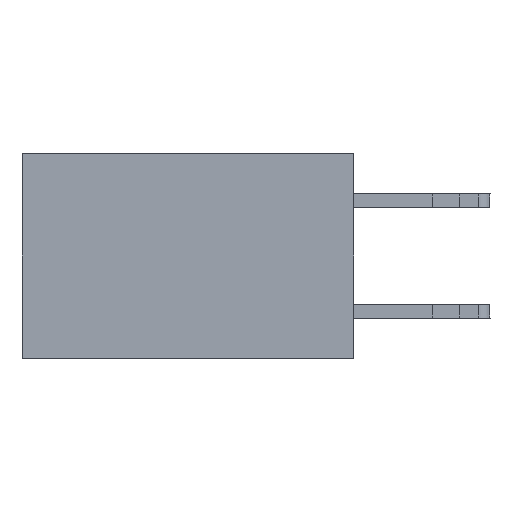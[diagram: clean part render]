
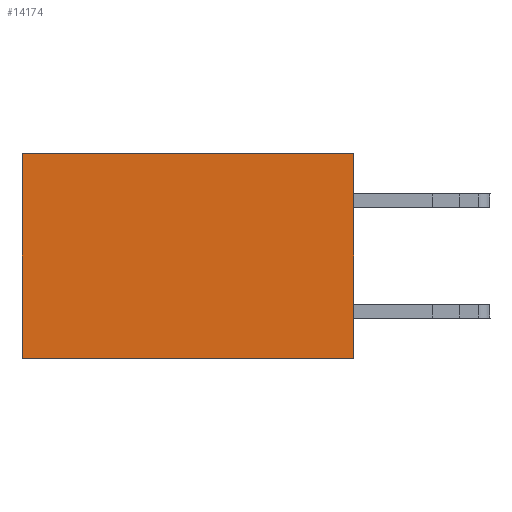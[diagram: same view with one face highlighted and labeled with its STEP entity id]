
A CAD part, left-side view. The second image highlights one B-rep face of the part: STEP entity #14174.
In plain terms, the highlighted planar face has unit normal (-1, 0, 0).
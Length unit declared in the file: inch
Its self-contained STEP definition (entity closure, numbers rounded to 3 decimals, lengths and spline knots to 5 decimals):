
#4 = DIRECTION ( 'NONE',  ( 0., 0., -1. ) ) ;
#76 = DIRECTION ( 'NONE',  ( 0., 1., 0. ) ) ;
#348 = VERTEX_POINT ( 'NONE', #5006 ) ;
#629 = LINE ( 'NONE', #1045, #10848 ) ;
#1045 = CARTESIAN_POINT ( 'NONE',  ( 0.2875, 0.6, 0. ) ) ;
#2003 = VERTEX_POINT ( 'NONE', #27059 ) ;
#3115 = VERTEX_POINT ( 'NONE', #6488 ) ;
#4076 = ORIENTED_EDGE ( 'NONE', *, *, #25145, .T. ) ;
#4203 = PLANE ( 'NONE',  #22888 ) ;
#5006 = CARTESIAN_POINT ( 'NONE',  ( 0.2875, 0., 0. ) ) ;
#5452 = CARTESIAN_POINT ( 'NONE',  ( 0.2875, 0., 0. ) ) ;
#6457 = LINE ( 'NONE', #21371, #27832 ) ;
#6488 = CARTESIAN_POINT ( 'NONE',  ( 0.2875, 0.6, -0.37 ) ) ;
#7638 = ORIENTED_EDGE ( 'NONE', *, *, #24230, .F. ) ;
#8536 = VERTEX_POINT ( 'NONE', #11412 ) ;
#9422 = ORIENTED_EDGE ( 'NONE', *, *, #11197, .F. ) ;
#10848 = VECTOR ( 'NONE', #14128, 39.37008 ) ;
#11197 = EDGE_CURVE ( 'NONE', #348, #2003, #12595, .T. ) ;
#11412 = CARTESIAN_POINT ( 'NONE',  ( 0.2875, 0.6, 0. ) ) ;
#12595 = LINE ( 'NONE', #5452, #26172 ) ;
#13113 = DIRECTION ( 'NONE',  ( 0., 0., -1. ) ) ;
#14128 = DIRECTION ( 'NONE',  ( 0., 0., -1. ) ) ;
#14174 = ADVANCED_FACE ( 'NONE', ( #24636 ), #4203, .F. ) ;
#15095 = CARTESIAN_POINT ( 'NONE',  ( 0.2875, 0., 0. ) ) ;
#17070 = VECTOR ( 'NONE', #20074, 39.37008 ) ;
#17993 = EDGE_CURVE ( 'NONE', #348, #8536, #27927, .T. ) ;
#19261 = DIRECTION ( 'NONE',  ( 1., 0., 0. ) ) ;
#20074 = DIRECTION ( 'NONE',  ( 0., 1., 0. ) ) ;
#20514 = EDGE_LOOP ( 'NONE', ( #4076, #7638, #9422, #22261 ) ) ;
#21371 = CARTESIAN_POINT ( 'NONE',  ( 0.2875, 0., -0.37 ) ) ;
#22261 = ORIENTED_EDGE ( 'NONE', *, *, #17993, .T. ) ;
#22263 = CARTESIAN_POINT ( 'NONE',  ( 0.2875, 0., 0. ) ) ;
#22888 = AXIS2_PLACEMENT_3D ( 'NONE', #15095, #19261, #13113 ) ;
#24230 = EDGE_CURVE ( 'NONE', #2003, #3115, #6457, .T. ) ;
#24636 = FACE_OUTER_BOUND ( 'NONE', #20514, .T. ) ;
#25145 = EDGE_CURVE ( 'NONE', #8536, #3115, #629, .T. ) ;
#26172 = VECTOR ( 'NONE', #4, 39.37008 ) ;
#27059 = CARTESIAN_POINT ( 'NONE',  ( 0.2875, 0., -0.37 ) ) ;
#27832 = VECTOR ( 'NONE', #76, 39.37008 ) ;
#27927 = LINE ( 'NONE', #22263, #17070 ) ;
